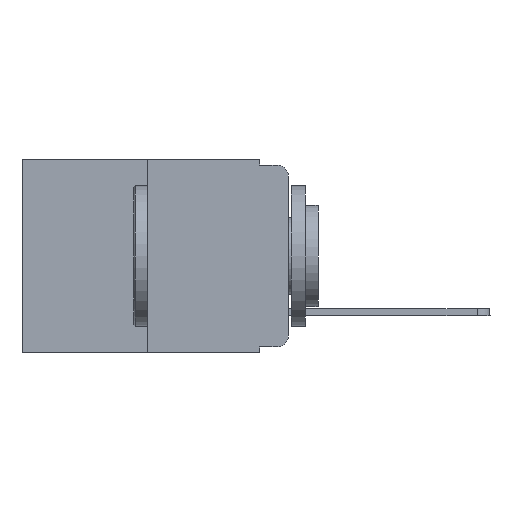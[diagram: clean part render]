
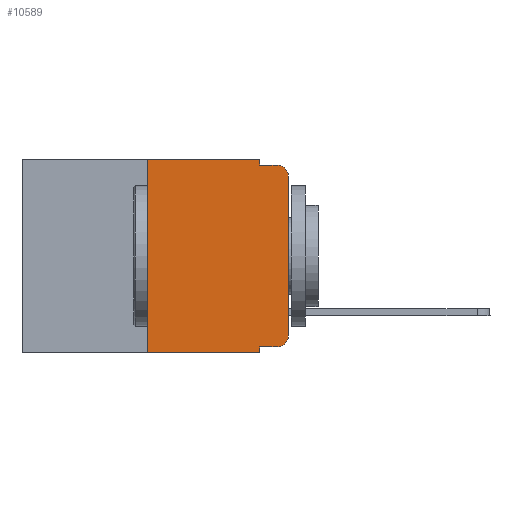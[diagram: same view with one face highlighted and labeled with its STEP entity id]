
A CAD part, left-side view. The second image highlights one B-rep face of the part: STEP entity #10589.
In plain terms, the highlighted planar face has unit normal (-1, 0, 0).
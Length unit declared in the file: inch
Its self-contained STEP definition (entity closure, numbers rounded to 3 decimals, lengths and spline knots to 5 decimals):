
#54 = VERTEX_POINT ( 'NONE', #16400 ) ;
#91 = VECTOR ( 'NONE', #10229, 39.37008 ) ;
#529 = VERTEX_POINT ( 'NONE', #7993 ) ;
#1125 = ORIENTED_EDGE ( 'NONE', *, *, #10982, .T. ) ;
#1301 = ORIENTED_EDGE ( 'NONE', *, *, #4635, .F. ) ;
#1515 = CARTESIAN_POINT ( 'NONE',  ( 0., 0.02, -0.01 ) ) ;
#1720 = VECTOR ( 'NONE', #12139, 39.37008 ) ;
#1887 = CARTESIAN_POINT ( 'NONE',  ( 0., 0.051, -0.333 ) ) ;
#1933 = CARTESIAN_POINT ( 'NONE',  ( 0., 0.02, -0.03 ) ) ;
#2190 = AXIS2_PLACEMENT_3D ( 'NONE', #5857, #13545, #13670 ) ;
#2278 = VECTOR ( 'NONE', #14366, 39.37008 ) ;
#2331 = VERTEX_POINT ( 'NONE', #10270 ) ;
#2340 = CARTESIAN_POINT ( 'NONE',  ( 0., 0.02, -0.313 ) ) ;
#2404 = EDGE_CURVE ( 'NONE', #12063, #7274, #12703, .T. ) ;
#2795 = VERTEX_POINT ( 'NONE', #10971 ) ;
#2960 = VERTEX_POINT ( 'NONE', #1515 ) ;
#3145 = DIRECTION ( 'NONE',  ( 0., 0., -1. ) ) ;
#3163 = LINE ( 'NONE', #8209, #3366 ) ;
#3366 = VECTOR ( 'NONE', #6770, 39.37008 ) ;
#3717 = ORIENTED_EDGE ( 'NONE', *, *, #2404, .T. ) ;
#3907 = CIRCLE ( 'NONE', #11008, 0.02 ) ;
#4143 = CARTESIAN_POINT ( 'NONE',  ( 0., 0., -0.03 ) ) ;
#4180 = CARTESIAN_POINT ( 'NONE',  ( 0., 0., 0. ) ) ;
#4365 = CARTESIAN_POINT ( 'NONE',  ( 0., 0.051, -0.01 ) ) ;
#4461 = LINE ( 'NONE', #4180, #2278 ) ;
#4635 = EDGE_CURVE ( 'NONE', #14525, #11290, #9019, .T. ) ;
#5274 = EDGE_CURVE ( 'NONE', #11290, #529, #6228, .T. ) ;
#5522 = DIRECTION ( 'NONE',  ( 0., -1., 0. ) ) ;
#5857 = CARTESIAN_POINT ( 'NONE',  ( 0., 0.473, 0. ) ) ;
#6015 = VECTOR ( 'NONE', #8819, 39.37008 ) ;
#6164 = CARTESIAN_POINT ( 'NONE',  ( 0., 0.473, -0.343 ) ) ;
#6228 = LINE ( 'NONE', #14251, #10795 ) ;
#6322 = VECTOR ( 'NONE', #15849, 39.37008 ) ;
#6554 = EDGE_CURVE ( 'NONE', #54, #14525, #3163, .T. ) ;
#6770 = DIRECTION ( 'NONE',  ( 0., 0., 1. ) ) ;
#6919 = CARTESIAN_POINT ( 'NONE',  ( 0., 0.02, -0.333 ) ) ;
#7091 = EDGE_LOOP ( 'NONE', ( #14075, #11515, #11265, #14170, #1301, #10772, #15170, #11023, #3717, #1125 ) ) ;
#7274 = VERTEX_POINT ( 'NONE', #6919 ) ;
#7430 = LINE ( 'NONE', #6164, #6015 ) ;
#7532 = EDGE_CURVE ( 'NONE', #12627, #2960, #3907, .T. ) ;
#7993 = CARTESIAN_POINT ( 'NONE',  ( 0., 0.051, -0.01 ) ) ;
#8106 = LINE ( 'NONE', #4365, #1720 ) ;
#8209 = CARTESIAN_POINT ( 'NONE',  ( 0., 0.25, 0. ) ) ;
#8524 = EDGE_CURVE ( 'NONE', #2795, #12627, #4461, .T. ) ;
#8819 = DIRECTION ( 'NONE',  ( 0., -1., 0. ) ) ;
#8838 = CARTESIAN_POINT ( 'NONE',  ( 0., 0.473, 0. ) ) ;
#9019 = LINE ( 'NONE', #8838, #91 ) ;
#9384 = DIRECTION ( 'NONE',  ( -1., 0., 0. ) ) ;
#9421 = CARTESIAN_POINT ( 'NONE',  ( 0., 0.051, 0. ) ) ;
#9780 = FACE_OUTER_BOUND ( 'NONE', #7091, .T. ) ;
#10229 = DIRECTION ( 'NONE',  ( 0., -1., 0. ) ) ;
#10270 = CARTESIAN_POINT ( 'NONE',  ( 0., 0.051, -0.343 ) ) ;
#10396 = EDGE_CURVE ( 'NONE', #54, #2331, #7430, .T. ) ;
#10589 = ADVANCED_FACE ( 'NONE', ( #9780 ), #10925, .F. ) ;
#10619 = DIRECTION ( 'NONE',  ( 0., 0., -1. ) ) ;
#10772 = ORIENTED_EDGE ( 'NONE', *, *, #6554, .F. ) ;
#10795 = VECTOR ( 'NONE', #10619, 39.37008 ) ;
#10925 = PLANE ( 'NONE',  #2190 ) ;
#10971 = CARTESIAN_POINT ( 'NONE',  ( 0., 0., -0.313 ) ) ;
#10982 = EDGE_CURVE ( 'NONE', #7274, #2795, #14163, .T. ) ;
#11008 = AXIS2_PLACEMENT_3D ( 'NONE', #1933, #9384, #3145 ) ;
#11023 = ORIENTED_EDGE ( 'NONE', *, *, #14073, .F. ) ;
#11265 = ORIENTED_EDGE ( 'NONE', *, *, #14706, .F. ) ;
#11290 = VERTEX_POINT ( 'NONE', #12639 ) ;
#11515 = ORIENTED_EDGE ( 'NONE', *, *, #7532, .T. ) ;
#11887 = DIRECTION ( 'NONE',  ( 0., 0., -1. ) ) ;
#12063 = VERTEX_POINT ( 'NONE', #1887 ) ;
#12139 = DIRECTION ( 'NONE',  ( 0., -1., 0. ) ) ;
#12627 = VERTEX_POINT ( 'NONE', #4143 ) ;
#12639 = CARTESIAN_POINT ( 'NONE',  ( 0., 0.051, 0. ) ) ;
#12703 = LINE ( 'NONE', #14282, #12905 ) ;
#12905 = VECTOR ( 'NONE', #5522, 39.37008 ) ;
#13100 = CARTESIAN_POINT ( 'NONE',  ( 0., 0.25, 0. ) ) ;
#13118 = DIRECTION ( 'NONE',  ( -1., 0., 0. ) ) ;
#13492 = LINE ( 'NONE', #9421, #6322 ) ;
#13545 = DIRECTION ( 'NONE',  ( 1., 0., 0. ) ) ;
#13670 = DIRECTION ( 'NONE',  ( 0., 0., -1. ) ) ;
#14073 = EDGE_CURVE ( 'NONE', #12063, #2331, #13492, .T. ) ;
#14075 = ORIENTED_EDGE ( 'NONE', *, *, #8524, .T. ) ;
#14139 = AXIS2_PLACEMENT_3D ( 'NONE', #2340, #13118, #11887 ) ;
#14163 = CIRCLE ( 'NONE', #14139, 0.02 ) ;
#14170 = ORIENTED_EDGE ( 'NONE', *, *, #5274, .F. ) ;
#14251 = CARTESIAN_POINT ( 'NONE',  ( 0., 0.051, 0. ) ) ;
#14282 = CARTESIAN_POINT ( 'NONE',  ( 0., 0.051, -0.333 ) ) ;
#14366 = DIRECTION ( 'NONE',  ( 0., 0., 1. ) ) ;
#14525 = VERTEX_POINT ( 'NONE', #13100 ) ;
#14706 = EDGE_CURVE ( 'NONE', #529, #2960, #8106, .T. ) ;
#15170 = ORIENTED_EDGE ( 'NONE', *, *, #10396, .T. ) ;
#15849 = DIRECTION ( 'NONE',  ( 0., 0., -1. ) ) ;
#16400 = CARTESIAN_POINT ( 'NONE',  ( 0., 0.25, -0.343 ) ) ;
